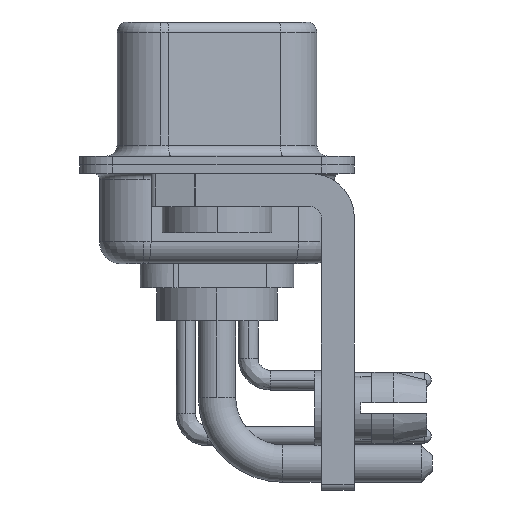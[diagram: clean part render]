
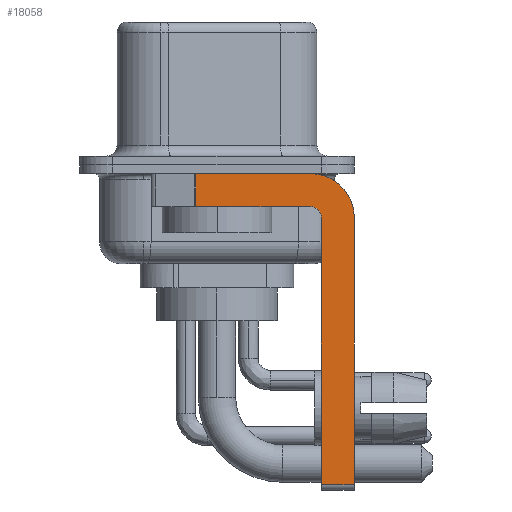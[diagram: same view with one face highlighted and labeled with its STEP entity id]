
A CAD part, left-side view. The second image highlights one B-rep face of the part: STEP entity #18058.
In plain terms, the highlighted planar face has unit normal (-1, 0, 0).
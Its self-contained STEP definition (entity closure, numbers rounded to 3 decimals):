
#55 = VERTEX_POINT ( 'NONE', #8231 ) ;
#657 = EDGE_CURVE ( 'NONE', #6881, #3287, #2017, .T. ) ;
#1721 = EDGE_LOOP ( 'NONE', ( #9766, #21052, #13904, #20661, #12284, #4067, #8593, #8107 ) ) ;
#1769 = CARTESIAN_POINT ( 'NONE',  ( -2.9, 0.978, -1.9 ) ) ;
#2017 = CIRCLE ( 'NONE', #22887, 2. ) ;
#2277 = LINE ( 'NONE', #14855, #21147 ) ;
#2955 = DIRECTION ( 'NONE',  ( 0., 0., -1. ) ) ;
#3287 = VERTEX_POINT ( 'NONE', #5551 ) ;
#3828 = EDGE_CURVE ( 'NONE', #55, #21547, #3877, .T. ) ;
#3877 = LINE ( 'NONE', #16663, #5926 ) ;
#4067 = ORIENTED_EDGE ( 'NONE', *, *, #11541, .T. ) ;
#4183 = CARTESIAN_POINT ( 'NONE',  ( -2.9, -4.25, -1.9 ) ) ;
#4471 = LINE ( 'NONE', #22169, #21981 ) ;
#4688 = CARTESIAN_POINT ( 'NONE',  ( -2.9, -4.25, -14.55 ) ) ;
#5030 = VECTOR ( 'NONE', #20850, 1000. ) ;
#5551 = CARTESIAN_POINT ( 'NONE',  ( -2.9, -6.25, -2.4 ) ) ;
#5607 = LINE ( 'NONE', #4183, #8342 ) ;
#5926 = VECTOR ( 'NONE', #18574, 1000. ) ;
#6415 = LINE ( 'NONE', #8296, #10097 ) ;
#6620 = VERTEX_POINT ( 'NONE', #7853 ) ;
#6881 = VERTEX_POINT ( 'NONE', #21643 ) ;
#7058 = VERTEX_POINT ( 'NONE', #11269 ) ;
#7853 = CARTESIAN_POINT ( 'NONE',  ( -2.9, -6.25, -14.55 ) ) ;
#8036 = CIRCLE ( 'NONE', #21346, 0.5 ) ;
#8107 = ORIENTED_EDGE ( 'NONE', *, *, #657, .F. ) ;
#8218 = VERTEX_POINT ( 'NONE', #10124 ) ;
#8219 = DIRECTION ( 'NONE',  ( -1., 0., 0. ) ) ;
#8231 = CARTESIAN_POINT ( 'NONE',  ( -2.9, 0.978, -0.4 ) ) ;
#8296 = CARTESIAN_POINT ( 'NONE',  ( -2.9, -6.25, -2.4 ) ) ;
#8342 = VECTOR ( 'NONE', #11394, 1000. ) ;
#8441 = EDGE_CURVE ( 'NONE', #10620, #21547, #5607, .T. ) ;
#8593 = ORIENTED_EDGE ( 'NONE', *, *, #17507, .F. ) ;
#9766 = ORIENTED_EDGE ( 'NONE', *, *, #21846, .F. ) ;
#9872 = DIRECTION ( 'NONE',  ( 0., 0., -1. ) ) ;
#10097 = VECTOR ( 'NONE', #9872, 1000. ) ;
#10124 = CARTESIAN_POINT ( 'NONE',  ( -2.9, -4.75, -2.4 ) ) ;
#10253 = DIRECTION ( 'NONE',  ( 0., 0., 1. ) ) ;
#10419 = PLANE ( 'NONE',  #10871 ) ;
#10620 = VERTEX_POINT ( 'NONE', #21776 ) ;
#10871 = AXIS2_PLACEMENT_3D ( 'NONE', #17427, #19694, #2955 ) ;
#11269 = CARTESIAN_POINT ( 'NONE',  ( -2.9, -4.75, -14.55 ) ) ;
#11394 = DIRECTION ( 'NONE',  ( 0., 1., 0. ) ) ;
#11541 = EDGE_CURVE ( 'NONE', #7058, #6620, #17500, .T. ) ;
#11568 = EDGE_CURVE ( 'NONE', #8218, #10620, #8036, .T. ) ;
#12284 = ORIENTED_EDGE ( 'NONE', *, *, #18741, .F. ) ;
#13904 = ORIENTED_EDGE ( 'NONE', *, *, #8441, .F. ) ;
#14855 = CARTESIAN_POINT ( 'NONE',  ( -2.9, -4.75, -14.8 ) ) ;
#16251 = DIRECTION ( 'NONE',  ( 0., 0., -1. ) ) ;
#16663 = CARTESIAN_POINT ( 'NONE',  ( -2.9, 0.978, -1.9 ) ) ;
#17427 = CARTESIAN_POINT ( 'NONE',  ( -2.9, -4.25, -2.4 ) ) ;
#17500 = LINE ( 'NONE', #4688, #5030 ) ;
#17507 = EDGE_CURVE ( 'NONE', #3287, #6620, #6415, .T. ) ;
#18058 = ADVANCED_FACE ( 'NONE', ( #19573 ), #10419, .F. ) ;
#18315 = DIRECTION ( 'NONE',  ( 0., 0., 1. ) ) ;
#18574 = DIRECTION ( 'NONE',  ( 0., 0., -1. ) ) ;
#18741 = EDGE_CURVE ( 'NONE', #7058, #8218, #2277, .T. ) ;
#19480 = DIRECTION ( 'NONE',  ( 1., 0., 0. ) ) ;
#19573 = FACE_OUTER_BOUND ( 'NONE', #1721, .T. ) ;
#19694 = DIRECTION ( 'NONE',  ( 1., 0., 0. ) ) ;
#20379 = DIRECTION ( 'NONE',  ( 0., -1., 0. ) ) ;
#20661 = ORIENTED_EDGE ( 'NONE', *, *, #11568, .F. ) ;
#20850 = DIRECTION ( 'NONE',  ( 0., -1., 0. ) ) ;
#21052 = ORIENTED_EDGE ( 'NONE', *, *, #3828, .T. ) ;
#21147 = VECTOR ( 'NONE', #18315, 1000. ) ;
#21346 = AXIS2_PLACEMENT_3D ( 'NONE', #23096, #8219, #10253 ) ;
#21547 = VERTEX_POINT ( 'NONE', #1769 ) ;
#21643 = CARTESIAN_POINT ( 'NONE',  ( -2.9, -4.25, -0.4 ) ) ;
#21776 = CARTESIAN_POINT ( 'NONE',  ( -2.9, -4.25, -1.9 ) ) ;
#21846 = EDGE_CURVE ( 'NONE', #55, #6881, #4471, .T. ) ;
#21981 = VECTOR ( 'NONE', #20379, 1000. ) ;
#22169 = CARTESIAN_POINT ( 'NONE',  ( -2.9, 3., -0.4 ) ) ;
#22887 = AXIS2_PLACEMENT_3D ( 'NONE', #23170, #19480, #16251 ) ;
#23096 = CARTESIAN_POINT ( 'NONE',  ( -2.9, -4.25, -2.4 ) ) ;
#23170 = CARTESIAN_POINT ( 'NONE',  ( -2.9, -4.25, -2.4 ) ) ;
